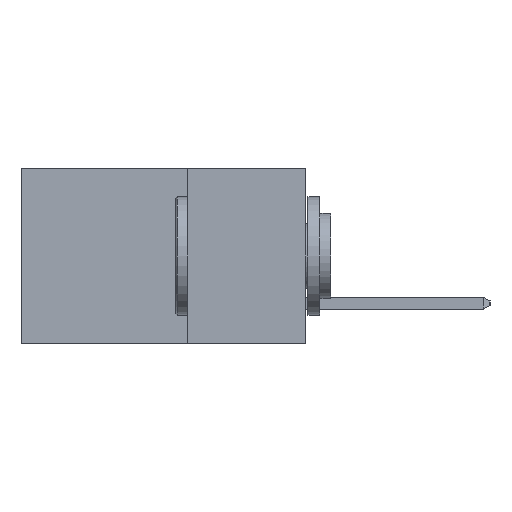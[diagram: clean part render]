
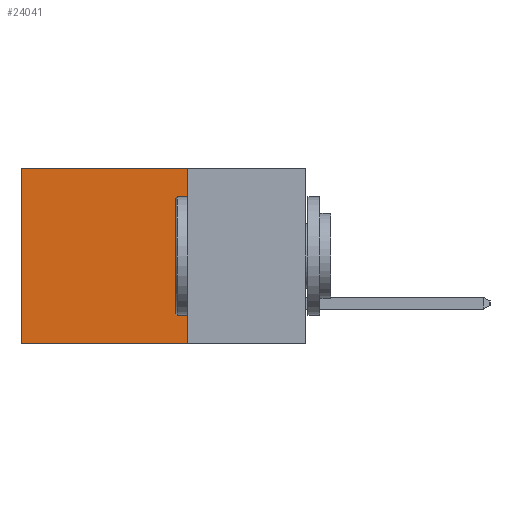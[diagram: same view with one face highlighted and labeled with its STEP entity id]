
A CAD part, left-side view. The second image highlights one B-rep face of the part: STEP entity #24041.
In plain terms, the highlighted planar face has unit normal (-1, 0, 0).
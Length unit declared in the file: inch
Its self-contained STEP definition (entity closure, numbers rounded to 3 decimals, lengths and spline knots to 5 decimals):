
#495 = DIRECTION ( 'NONE',  ( 0., 0., -1. ) ) ;
#552 = VERTEX_POINT ( 'NONE', #1173 ) ;
#1098 = DIRECTION ( 'NONE',  ( 0., 1., 0. ) ) ;
#1173 = CARTESIAN_POINT ( 'NONE',  ( 0.298, 0.25, 0. ) ) ;
#1897 = CARTESIAN_POINT ( 'NONE',  ( 0.298, 0.6, 0. ) ) ;
#2020 = LINE ( 'NONE', #15524, #2689 ) ;
#2645 = ORIENTED_EDGE ( 'NONE', *, *, #21065, .F. ) ;
#2689 = VECTOR ( 'NONE', #495, 39.37008 ) ;
#3320 = LINE ( 'NONE', #13832, #18378 ) ;
#3954 = ORIENTED_EDGE ( 'NONE', *, *, #15185, .T. ) ;
#5197 = VECTOR ( 'NONE', #14739, 39.37008 ) ;
#6327 = LINE ( 'NONE', #17939, #22635 ) ;
#6705 = CARTESIAN_POINT ( 'NONE',  ( 0.298, 0.6, 0. ) ) ;
#7084 = FACE_OUTER_BOUND ( 'NONE', #26088, .T. ) ;
#7482 = CARTESIAN_POINT ( 'NONE',  ( 0.298, 0.25, -0.37 ) ) ;
#8093 = CARTESIAN_POINT ( 'NONE',  ( 0.298, 0.6, -0.37 ) ) ;
#10258 = DIRECTION ( 'NONE',  ( 0., 0., -1. ) ) ;
#10849 = LINE ( 'NONE', #1897, #5197 ) ;
#11850 = EDGE_CURVE ( 'NONE', #24211, #14488, #10849, .T. ) ;
#13832 = CARTESIAN_POINT ( 'NONE',  ( 0.298, 0.25, 0. ) ) ;
#14112 = ORIENTED_EDGE ( 'NONE', *, *, #19125, .F. ) ;
#14488 = VERTEX_POINT ( 'NONE', #8093 ) ;
#14739 = DIRECTION ( 'NONE',  ( 0., 0., -1. ) ) ;
#15172 = VERTEX_POINT ( 'NONE', #7482 ) ;
#15185 = EDGE_CURVE ( 'NONE', #552, #24211, #3320, .T. ) ;
#15524 = CARTESIAN_POINT ( 'NONE',  ( 0.298, 0.25, 0. ) ) ;
#15794 = ORIENTED_EDGE ( 'NONE', *, *, #11850, .T. ) ;
#17939 = CARTESIAN_POINT ( 'NONE',  ( 0.298, 0.25, -0.37 ) ) ;
#18378 = VECTOR ( 'NONE', #1098, 39.37008 ) ;
#18725 = CARTESIAN_POINT ( 'NONE',  ( 0.298, 0.25, 0. ) ) ;
#19125 = EDGE_CURVE ( 'NONE', #552, #15172, #2020, .T. ) ;
#20953 = PLANE ( 'NONE',  #23948 ) ;
#21065 = EDGE_CURVE ( 'NONE', #15172, #14488, #6327, .T. ) ;
#22635 = VECTOR ( 'NONE', #25866, 39.37008 ) ;
#23047 = DIRECTION ( 'NONE',  ( 1., 0., 0. ) ) ;
#23948 = AXIS2_PLACEMENT_3D ( 'NONE', #18725, #23047, #10258 ) ;
#24041 = ADVANCED_FACE ( 'NONE', ( #7084 ), #20953, .F. ) ;
#24211 = VERTEX_POINT ( 'NONE', #6705 ) ;
#25866 = DIRECTION ( 'NONE',  ( 0., 1., 0. ) ) ;
#26088 = EDGE_LOOP ( 'NONE', ( #15794, #2645, #14112, #3954 ) ) ;
